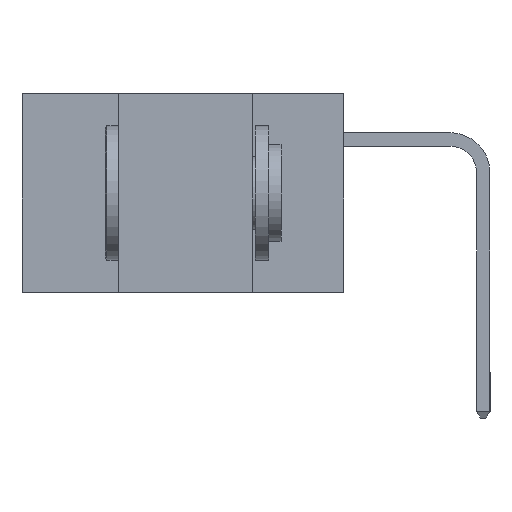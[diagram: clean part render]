
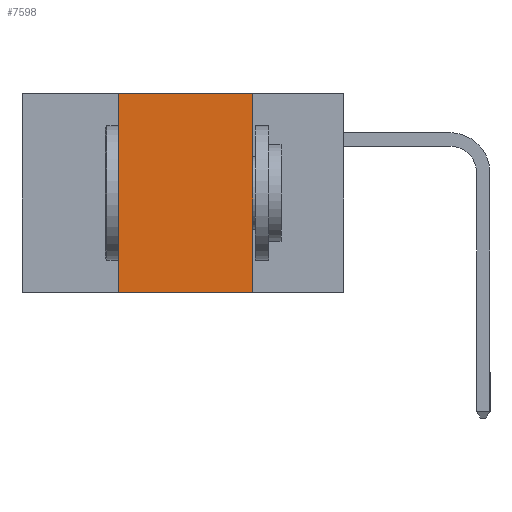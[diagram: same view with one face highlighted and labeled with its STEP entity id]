
A CAD part, left-side view. The second image highlights one B-rep face of the part: STEP entity #7598.
In plain terms, the highlighted planar face has unit normal (-1, 0, 0).
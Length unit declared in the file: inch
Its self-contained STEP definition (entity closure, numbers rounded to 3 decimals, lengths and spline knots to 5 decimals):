
#77 = LINE ( 'NONE', #7154, #361 ) ;
#361 = VECTOR ( 'NONE', #3900, 39.37008 ) ;
#952 = VERTEX_POINT ( 'NONE', #4594 ) ;
#1362 = CARTESIAN_POINT ( 'NONE',  ( 0., 0.17, -0.37 ) ) ;
#1656 = ORIENTED_EDGE ( 'NONE', *, *, #10979, .F. ) ;
#1991 = PLANE ( 'NONE',  #2628 ) ;
#2029 = CARTESIAN_POINT ( 'NONE',  ( 0., 0.6, 0. ) ) ;
#2163 = VECTOR ( 'NONE', #2894, 39.37008 ) ;
#2628 = AXIS2_PLACEMENT_3D ( 'NONE', #2029, #8000, #4458 ) ;
#2745 = VERTEX_POINT ( 'NONE', #1362 ) ;
#2800 = DIRECTION ( 'NONE',  ( 0., -1., 0. ) ) ;
#2894 = DIRECTION ( 'NONE',  ( 0., 0., 1. ) ) ;
#3115 = DIRECTION ( 'NONE',  ( 0., 0., -1. ) ) ;
#3356 = LINE ( 'NONE', #7966, #8907 ) ;
#3900 = DIRECTION ( 'NONE',  ( 0., -1., 0. ) ) ;
#3989 = CARTESIAN_POINT ( 'NONE',  ( 0., 0.17, 0. ) ) ;
#4458 = DIRECTION ( 'NONE',  ( 0., 0., -1. ) ) ;
#4532 = VERTEX_POINT ( 'NONE', #6545 ) ;
#4594 = CARTESIAN_POINT ( 'NONE',  ( 0., 0.42, -0.37 ) ) ;
#4699 = CARTESIAN_POINT ( 'NONE',  ( 0., 0.42, 0. ) ) ;
#4863 = ORIENTED_EDGE ( 'NONE', *, *, #10456, .F. ) ;
#5516 = VERTEX_POINT ( 'NONE', #8810 ) ;
#6218 = LINE ( 'NONE', #4699, #2163 ) ;
#6236 = EDGE_CURVE ( 'NONE', #952, #2745, #77, .T. ) ;
#6529 = FACE_OUTER_BOUND ( 'NONE', #9840, .T. ) ;
#6545 = CARTESIAN_POINT ( 'NONE',  ( 0., 0.17, 0. ) ) ;
#6628 = ORIENTED_EDGE ( 'NONE', *, *, #10311, .F. ) ;
#6723 = VECTOR ( 'NONE', #3115, 39.37008 ) ;
#7139 = LINE ( 'NONE', #3989, #6723 ) ;
#7154 = CARTESIAN_POINT ( 'NONE',  ( 0., 0.6, -0.37 ) ) ;
#7598 = ADVANCED_FACE ( 'NONE', ( #6529 ), #1991, .F. ) ;
#7966 = CARTESIAN_POINT ( 'NONE',  ( 0., 0.6, 0. ) ) ;
#8000 = DIRECTION ( 'NONE',  ( 1., 0., 0. ) ) ;
#8465 = ORIENTED_EDGE ( 'NONE', *, *, #6236, .T. ) ;
#8810 = CARTESIAN_POINT ( 'NONE',  ( 0., 0.42, 0. ) ) ;
#8907 = VECTOR ( 'NONE', #2800, 39.37008 ) ;
#9840 = EDGE_LOOP ( 'NONE', ( #4863, #1656, #6628, #8465 ) ) ;
#10311 = EDGE_CURVE ( 'NONE', #952, #5516, #6218, .T. ) ;
#10456 = EDGE_CURVE ( 'NONE', #4532, #2745, #7139, .T. ) ;
#10979 = EDGE_CURVE ( 'NONE', #5516, #4532, #3356, .T. ) ;
